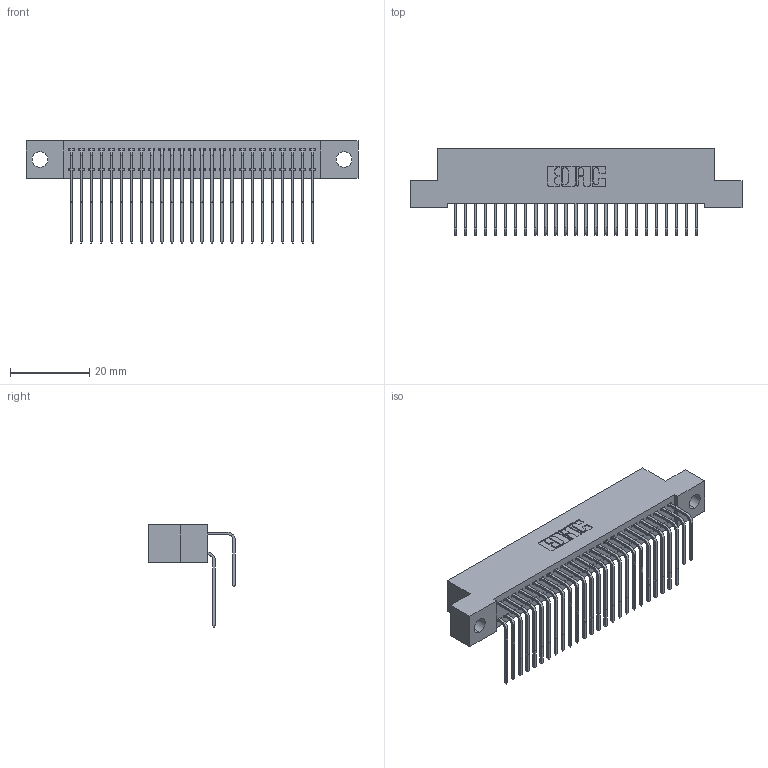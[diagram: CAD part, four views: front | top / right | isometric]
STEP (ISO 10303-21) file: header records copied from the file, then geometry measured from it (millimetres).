
FILE_DESCRIPTION (( 'STEP AP203' ), '1' );
FILE_NAME ('392-050-558-204.STEP', '2019-10-08T11:41:38', ( '' ), ( '' ), 'SwSTEP 2.0', 'SolidWorks 2016', '' );
FILE_SCHEMA (( 'CONFIG_CONTROL_DESIGN' ));
Length unit declared in the file: inch
Products named in the file (4): 342 Part_.156 TH; 345-292-001_558 559 Tail - 1; 345-292-001_558 Tail - 2; 392-050-558-204
Assembly tree (51 placements, depth 2):
  392-050-558-204
    342 Part_.156 TH
    345-292-001_558 559 Tail - 1  x25
    345-292-001_558 Tail - 2  x25
Bounding box: 83.82 x 21.91 x 25.78 mm (x, y, z)
Volume: 7652.2 mm3; surface area: 13165.9 mm2
Topology: 51 solids, 51 shells, 2810 faces, 8349 edges, 5498 vertices
Faces by surface type: plane 1966, cylinder 844
Entity records: 19937 total; most frequent: CARTESIAN_POINT 3373, ORIENTED_EDGE 3258, DIRECTION 2893, EDGE_CURVE 1629, LINE 1461, VECTOR 1461, VERTEX_POINT 1082, AXIS2_PLACEMENT_3D 716
